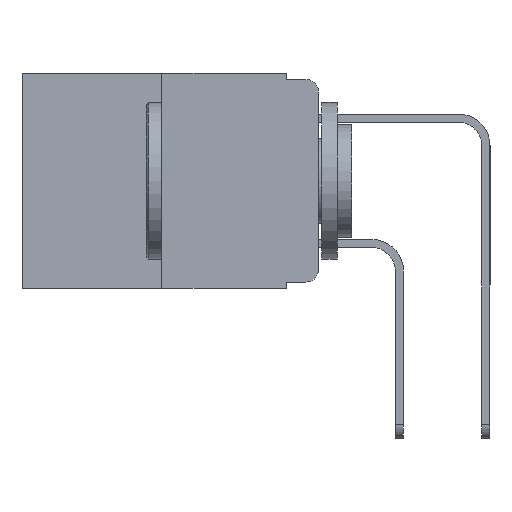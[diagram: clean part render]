
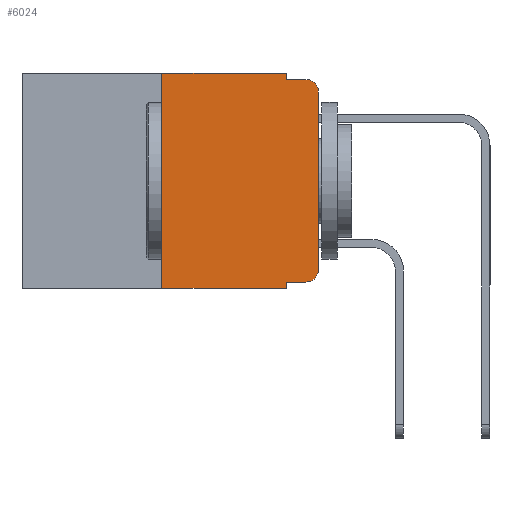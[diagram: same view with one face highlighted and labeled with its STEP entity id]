
A CAD part, left-side view. The second image highlights one B-rep face of the part: STEP entity #6024.
In plain terms, the highlighted planar face has unit normal (-1, 0, 0).
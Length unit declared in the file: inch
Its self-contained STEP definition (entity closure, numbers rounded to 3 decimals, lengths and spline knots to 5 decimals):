
#106 = ORIENTED_EDGE ( 'NONE', *, *, #13735, .F. ) ;
#190 = VECTOR ( 'NONE', #7809, 39.37008 ) ;
#979 = CARTESIAN_POINT ( 'NONE',  ( 0., 0.02, -0.333 ) ) ;
#1038 = CARTESIAN_POINT ( 'NONE',  ( 0., 0.25, -0.343 ) ) ;
#1183 = CARTESIAN_POINT ( 'NONE',  ( 0., 0.25, 0. ) ) ;
#1605 = VECTOR ( 'NONE', #10311, 39.37008 ) ;
#1850 = CARTESIAN_POINT ( 'NONE',  ( 0., 0.02, -0.313 ) ) ;
#2007 = AXIS2_PLACEMENT_3D ( 'NONE', #1850, #11708, #3428 ) ;
#2130 = VECTOR ( 'NONE', #6491, 39.37008 ) ;
#2260 = ORIENTED_EDGE ( 'NONE', *, *, #15102, .T. ) ;
#3007 = EDGE_CURVE ( 'NONE', #6245, #14947, #10577, .T. ) ;
#3155 = CARTESIAN_POINT ( 'NONE',  ( 0., 0.02, -0.03 ) ) ;
#3292 = CARTESIAN_POINT ( 'NONE',  ( 0., 0.473, 0. ) ) ;
#3428 = DIRECTION ( 'NONE',  ( 0., 0., -1. ) ) ;
#3850 = LINE ( 'NONE', #6557, #17941 ) ;
#3968 = ORIENTED_EDGE ( 'NONE', *, *, #13985, .F. ) ;
#4072 = VERTEX_POINT ( 'NONE', #17232 ) ;
#4079 = EDGE_CURVE ( 'NONE', #17800, #4072, #5688, .T. ) ;
#4160 = VECTOR ( 'NONE', #17191, 39.37008 ) ;
#4281 = LINE ( 'NONE', #15891, #7541 ) ;
#4694 = DIRECTION ( 'NONE',  ( 0., 0., -1. ) ) ;
#4740 = CARTESIAN_POINT ( 'NONE',  ( 0., 0.02, -0.01 ) ) ;
#4959 = DIRECTION ( 'NONE',  ( 0., 0., -1. ) ) ;
#5202 = CARTESIAN_POINT ( 'NONE',  ( 0., 0.051, -0.343 ) ) ;
#5219 = VERTEX_POINT ( 'NONE', #11028 ) ;
#5382 = AXIS2_PLACEMENT_3D ( 'NONE', #3292, #17042, #8941 ) ;
#5688 = LINE ( 'NONE', #14549, #2130 ) ;
#6024 = ADVANCED_FACE ( 'NONE', ( #13628 ), #15681, .F. ) ;
#6128 = CARTESIAN_POINT ( 'NONE',  ( 0., 0., -0.03 ) ) ;
#6140 = CIRCLE ( 'NONE', #13930, 0.02 ) ;
#6245 = VERTEX_POINT ( 'NONE', #7916 ) ;
#6491 = DIRECTION ( 'NONE',  ( 0., -1., 0. ) ) ;
#6557 = CARTESIAN_POINT ( 'NONE',  ( 0., 0.051, 0. ) ) ;
#6668 = ORIENTED_EDGE ( 'NONE', *, *, #17285, .T. ) ;
#7541 = VECTOR ( 'NONE', #13165, 39.37008 ) ;
#7809 = DIRECTION ( 'NONE',  ( 0., 0., 1. ) ) ;
#7916 = CARTESIAN_POINT ( 'NONE',  ( 0., 0.051, -0.01 ) ) ;
#8104 = VERTEX_POINT ( 'NONE', #15558 ) ;
#8132 = ORIENTED_EDGE ( 'NONE', *, *, #15019, .T. ) ;
#8941 = DIRECTION ( 'NONE',  ( 0., 0., -1. ) ) ;
#8984 = CARTESIAN_POINT ( 'NONE',  ( 0., 0.473, -0.343 ) ) ;
#9174 = CARTESIAN_POINT ( 'NONE',  ( 0., 0., 0. ) ) ;
#10000 = ORIENTED_EDGE ( 'NONE', *, *, #16348, .T. ) ;
#10311 = DIRECTION ( 'NONE',  ( 0., -1., 0. ) ) ;
#10577 = LINE ( 'NONE', #17185, #4160 ) ;
#11028 = CARTESIAN_POINT ( 'NONE',  ( 0., 0.051, -0.333 ) ) ;
#11550 = LINE ( 'NONE', #9174, #190 ) ;
#11708 = DIRECTION ( 'NONE',  ( -1., 0., 0. ) ) ;
#11777 = VECTOR ( 'NONE', #4959, 39.37008 ) ;
#11904 = ORIENTED_EDGE ( 'NONE', *, *, #18063, .T. ) ;
#12108 = VERTEX_POINT ( 'NONE', #6128 ) ;
#12427 = DIRECTION ( 'NONE',  ( 0., 0., 1. ) ) ;
#12555 = ORIENTED_EDGE ( 'NONE', *, *, #17296, .F. ) ;
#12824 = LINE ( 'NONE', #8984, #1605 ) ;
#12834 = DIRECTION ( 'NONE',  ( -1., 0., 0. ) ) ;
#13165 = DIRECTION ( 'NONE',  ( 0., -1., 0. ) ) ;
#13628 = FACE_OUTER_BOUND ( 'NONE', #17692, .T. ) ;
#13699 = LINE ( 'NONE', #15155, #16890 ) ;
#13735 = EDGE_CURVE ( 'NONE', #4072, #6245, #3850, .T. ) ;
#13930 = AXIS2_PLACEMENT_3D ( 'NONE', #3155, #12834, #4694 ) ;
#13985 = EDGE_CURVE ( 'NONE', #14703, #17800, #13699, .T. ) ;
#14221 = ORIENTED_EDGE ( 'NONE', *, *, #3007, .F. ) ;
#14549 = CARTESIAN_POINT ( 'NONE',  ( 0., 0.473, 0. ) ) ;
#14703 = VERTEX_POINT ( 'NONE', #1038 ) ;
#14947 = VERTEX_POINT ( 'NONE', #4740 ) ;
#15019 = EDGE_CURVE ( 'NONE', #14703, #15921, #12824, .T. ) ;
#15102 = EDGE_CURVE ( 'NONE', #5219, #17710, #4281, .T. ) ;
#15155 = CARTESIAN_POINT ( 'NONE',  ( 0., 0.25, 0. ) ) ;
#15400 = LINE ( 'NONE', #17106, #11777 ) ;
#15558 = CARTESIAN_POINT ( 'NONE',  ( 0., 0., -0.313 ) ) ;
#15681 = PLANE ( 'NONE',  #5382 ) ;
#15891 = CARTESIAN_POINT ( 'NONE',  ( 0., 0.051, -0.333 ) ) ;
#15921 = VERTEX_POINT ( 'NONE', #5202 ) ;
#16254 = CIRCLE ( 'NONE', #2007, 0.02 ) ;
#16348 = EDGE_CURVE ( 'NONE', #12108, #14947, #6140, .T. ) ;
#16789 = ORIENTED_EDGE ( 'NONE', *, *, #4079, .F. ) ;
#16890 = VECTOR ( 'NONE', #12427, 39.37008 ) ;
#17042 = DIRECTION ( 'NONE',  ( 1., 0., 0. ) ) ;
#17106 = CARTESIAN_POINT ( 'NONE',  ( 0., 0.051, 0. ) ) ;
#17185 = CARTESIAN_POINT ( 'NONE',  ( 0., 0.051, -0.01 ) ) ;
#17191 = DIRECTION ( 'NONE',  ( 0., -1., 0. ) ) ;
#17232 = CARTESIAN_POINT ( 'NONE',  ( 0., 0.051, 0. ) ) ;
#17285 = EDGE_CURVE ( 'NONE', #17710, #8104, #16254, .T. ) ;
#17296 = EDGE_CURVE ( 'NONE', #5219, #15921, #15400, .T. ) ;
#17347 = DIRECTION ( 'NONE',  ( 0., 0., -1. ) ) ;
#17692 = EDGE_LOOP ( 'NONE', ( #11904, #10000, #14221, #106, #16789, #3968, #8132, #12555, #2260, #6668 ) ) ;
#17710 = VERTEX_POINT ( 'NONE', #979 ) ;
#17800 = VERTEX_POINT ( 'NONE', #1183 ) ;
#17941 = VECTOR ( 'NONE', #17347, 39.37008 ) ;
#18063 = EDGE_CURVE ( 'NONE', #8104, #12108, #11550, .T. ) ;
